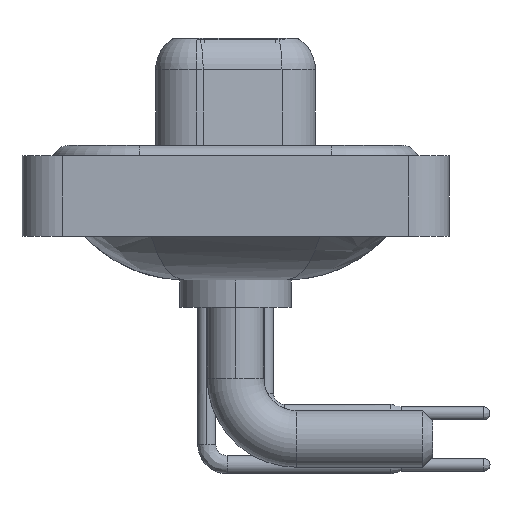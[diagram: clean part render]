
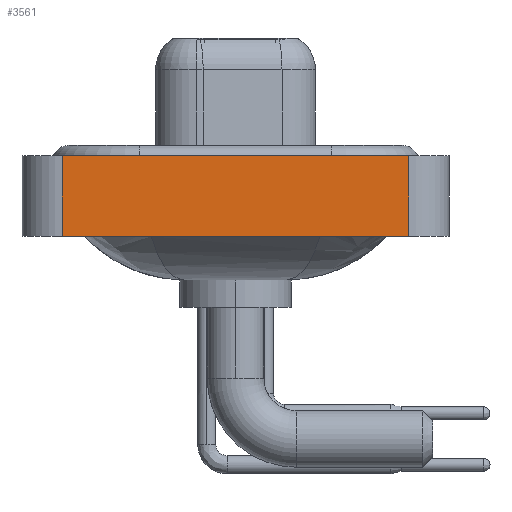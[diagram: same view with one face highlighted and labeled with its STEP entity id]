
A CAD part, left-side view. The second image highlights one B-rep face of the part: STEP entity #3561.
In plain terms, the highlighted planar face has unit normal (-1, 0, 0).
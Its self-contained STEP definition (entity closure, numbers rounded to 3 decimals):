
#445 = VERTEX_POINT ( 'NONE', #9739 ) ;
#767 = VECTOR ( 'NONE', #5296, 1000. ) ;
#1157 = AXIS2_PLACEMENT_3D ( 'NONE', #9159, #12504, #7688 ) ;
#1389 = ORIENTED_EDGE ( 'NONE', *, *, #13816, .T. ) ;
#2120 = DIRECTION ( 'NONE',  ( 0., 0., 1. ) ) ;
#2526 = EDGE_CURVE ( 'NONE', #6652, #445, #6942, .T. ) ;
#3561 = ADVANCED_FACE ( 'NONE', ( #17918 ), #12973, .T. ) ;
#5104 = CARTESIAN_POINT ( 'NONE',  ( -7.35, -8.55, -3.6 ) ) ;
#5296 = DIRECTION ( 'NONE',  ( 0., -1., 0. ) ) ;
#5891 = VECTOR ( 'NONE', #11003, 1000. ) ;
#5920 = LINE ( 'NONE', #16134, #22076 ) ;
#6652 = VERTEX_POINT ( 'NONE', #21891 ) ;
#6942 = LINE ( 'NONE', #19583, #17194 ) ;
#7014 = CARTESIAN_POINT ( 'NONE',  ( -7.35, -8.55, -3.6 ) ) ;
#7184 = ORIENTED_EDGE ( 'NONE', *, *, #2526, .F. ) ;
#7411 = EDGE_LOOP ( 'NONE', ( #16851, #11655, #7184, #1389 ) ) ;
#7688 = DIRECTION ( 'NONE',  ( 0., 0., 1. ) ) ;
#9159 = CARTESIAN_POINT ( 'NONE',  ( -7.35, -8.55, -3.6 ) ) ;
#9739 = CARTESIAN_POINT ( 'NONE',  ( -7.35, 8.55, 0.4 ) ) ;
#10226 = LINE ( 'NONE', #7014, #767 ) ;
#11003 = DIRECTION ( 'NONE',  ( 0., 0., 1. ) ) ;
#11655 = ORIENTED_EDGE ( 'NONE', *, *, #18603, .F. ) ;
#12504 = DIRECTION ( 'NONE',  ( -1., 0., 0. ) ) ;
#12576 = VERTEX_POINT ( 'NONE', #17235 ) ;
#12855 = CARTESIAN_POINT ( 'NONE',  ( -7.35, -8.55, -3.6 ) ) ;
#12921 = DIRECTION ( 'NONE',  ( 0., -1., 0. ) ) ;
#12973 = PLANE ( 'NONE',  #1157 ) ;
#13816 = EDGE_CURVE ( 'NONE', #6652, #21699, #10226, .T. ) ;
#14068 = EDGE_CURVE ( 'NONE', #21699, #12576, #14460, .T. ) ;
#14460 = LINE ( 'NONE', #12855, #5891 ) ;
#16134 = CARTESIAN_POINT ( 'NONE',  ( -7.35, -8.55, 0.4 ) ) ;
#16851 = ORIENTED_EDGE ( 'NONE', *, *, #14068, .T. ) ;
#17194 = VECTOR ( 'NONE', #2120, 1000. ) ;
#17235 = CARTESIAN_POINT ( 'NONE',  ( -7.35, -8.55, 0.4 ) ) ;
#17918 = FACE_OUTER_BOUND ( 'NONE', #7411, .T. ) ;
#18603 = EDGE_CURVE ( 'NONE', #445, #12576, #5920, .T. ) ;
#19583 = CARTESIAN_POINT ( 'NONE',  ( -7.35, 8.55, -3.6 ) ) ;
#21699 = VERTEX_POINT ( 'NONE', #5104 ) ;
#21891 = CARTESIAN_POINT ( 'NONE',  ( -7.35, 8.55, -3.6 ) ) ;
#22076 = VECTOR ( 'NONE', #12921, 1000. ) ;
